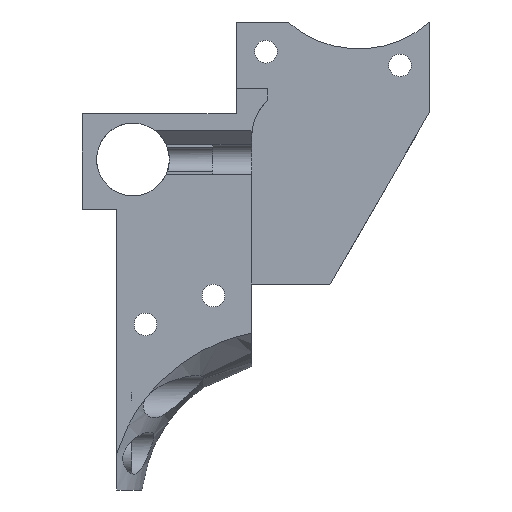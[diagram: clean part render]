
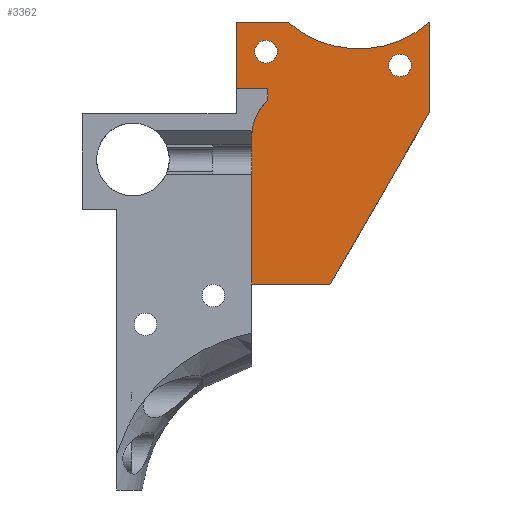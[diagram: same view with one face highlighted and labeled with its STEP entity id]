
A CAD part, left-side view. The second image highlights one B-rep face of the part: STEP entity #3362.
In plain terms, the highlighted planar face has unit normal (-1, 0, 0).
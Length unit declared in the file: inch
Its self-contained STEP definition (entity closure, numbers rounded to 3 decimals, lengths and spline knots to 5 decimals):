
#197=FACE_BOUND('',#874,.T.);
#198=FACE_BOUND('',#875,.T.);
#223=CIRCLE('',#3423,0.25);
#228=CIRCLE('',#3508,0.05906);
#230=CIRCLE('',#3511,0.05906);
#233=CIRCLE('',#3515,0.559);
#675=FACE_OUTER_BOUND('',#873,.T.);
#873=EDGE_LOOP('',(#3140,#3141,#3142,#3143,#3144,#3145,#3146,#3147,#3148,
#3149));
#874=EDGE_LOOP('',(#3150));
#875=EDGE_LOOP('',(#3151));
#914=LINE('',#4498,#1110);
#1031=LINE('',#5590,#1227);
#1041=LINE('',#9068,#1237);
#1048=LINE('',#9093,#1244);
#1049=LINE('',#9095,#1245);
#1068=LINE('',#9408,#1264);
#1070=LINE('',#9411,#1266);
#1071=LINE('',#9413,#1267);
#1110=VECTOR('',#3688,0.3937);
#1227=VECTOR('',#3821,0.3937);
#1237=VECTOR('',#3977,0.3937);
#1244=VECTOR('',#4004,0.3937);
#1245=VECTOR('',#4007,0.3937);
#1264=VECTOR('',#4084,0.3937);
#1266=VECTOR('',#4088,0.3937);
#1267=VECTOR('',#4091,0.3937);
#1325=VERTEX_POINT('',#4483);
#1326=VERTEX_POINT('',#4485);
#1330=VERTEX_POINT('',#4496);
#1551=VERTEX_POINT('',#5587);
#1552=VERTEX_POINT('',#5589);
#1590=VERTEX_POINT('',#9067);
#1591=VERTEX_POINT('',#9071);
#1593=VERTEX_POINT('',#9077);
#1597=VERTEX_POINT('',#9086);
#1598=VERTEX_POINT('',#9088);
#1608=VERTEX_POINT('',#9405);
#1609=VERTEX_POINT('',#9407);
#1683=EDGE_CURVE('',#1326,#1325,#223,.T.);
#1690=EDGE_CURVE('',#1325,#1330,#914,.T.);
#1916=EDGE_CURVE('',#1551,#1552,#1031,.T.);
#2066=EDGE_CURVE('',#1326,#1590,#1041,.T.);
#2068=EDGE_CURVE('',#1591,#1591,#228,.T.);
#2071=EDGE_CURVE('',#1593,#1593,#230,.T.);
#2076=EDGE_CURVE('',#1597,#1598,#233,.T.);
#2079=EDGE_CURVE('',#1552,#1597,#1048,.T.);
#2080=EDGE_CURVE('',#1590,#1551,#1049,.T.);
#2120=EDGE_CURVE('',#1609,#1608,#1068,.T.);
#2122=EDGE_CURVE('',#1330,#1609,#1070,.T.);
#2123=EDGE_CURVE('',#1608,#1598,#1071,.T.);
#3140=ORIENTED_EDGE('',*,*,#1683,.T.);
#3141=ORIENTED_EDGE('',*,*,#1690,.T.);
#3142=ORIENTED_EDGE('',*,*,#2122,.T.);
#3143=ORIENTED_EDGE('',*,*,#2120,.T.);
#3144=ORIENTED_EDGE('',*,*,#2123,.T.);
#3145=ORIENTED_EDGE('',*,*,#2076,.F.);
#3146=ORIENTED_EDGE('',*,*,#2079,.F.);
#3147=ORIENTED_EDGE('',*,*,#1916,.F.);
#3148=ORIENTED_EDGE('',*,*,#2080,.F.);
#3149=ORIENTED_EDGE('',*,*,#2066,.F.);
#3150=ORIENTED_EDGE('',*,*,#2068,.T.);
#3151=ORIENTED_EDGE('',*,*,#2071,.T.);
#3185=PLANE('',#3549);
#3362=ADVANCED_FACE('',(#675,#197,#198),#3185,.T.);
#3423=AXIS2_PLACEMENT_3D('',#4486,#3677,#3678);
#3508=AXIS2_PLACEMENT_3D('',#9072,#3981,#3982);
#3511=AXIS2_PLACEMENT_3D('',#9078,#3988,#3989);
#3515=AXIS2_PLACEMENT_3D('',#9089,#3998,#3999);
#3549=AXIS2_PLACEMENT_3D('',#9414,#4092,#4093);
#3677=DIRECTION('center_axis',(-1.,0.,0.));
#3678=DIRECTION('ref_axis',(0.,0.707,0.707));
#3688=DIRECTION('',(0.,0.,-1.));
#3821=DIRECTION('',(0.,0.,1.));
#3977=DIRECTION('',(0.,0.,1.));
#3981=DIRECTION('center_axis',(1.,0.,0.));
#3982=DIRECTION('ref_axis',(0.,0.,1.));
#3988=DIRECTION('center_axis',(1.,0.,0.));
#3989=DIRECTION('ref_axis',(0.,0.,1.));
#3998=DIRECTION('center_axis',(-1.,0.,0.));
#3999=DIRECTION('ref_axis',(0.,1.,0.));
#4004=DIRECTION('',(0.,-1.,0.));
#4007=DIRECTION('',(0.,1.,0.));
#4084=DIRECTION('',(0.,-0.5,0.866));
#4088=DIRECTION('',(0.,-1.,0.));
#4091=DIRECTION('',(0.,0.,1.));
#4092=DIRECTION('center_axis',(-1.,0.,0.));
#4093=DIRECTION('ref_axis',(0.,0.,1.));
#4483=CARTESIAN_POINT('',(-0.1875,-1.335,-2.188));
#4485=CARTESIAN_POINT('',(-0.1875,-1.4195,-2.00062));
#4486=CARTESIAN_POINT('Origin',(-0.1875,-1.585,-2.188));
#4496=CARTESIAN_POINT('',(-0.1875,-1.335,-2.963));
#4498=CARTESIAN_POINT('',(-0.1875,-1.335,-2.70675));
#5587=CARTESIAN_POINT('',(-0.1875,-1.254,-1.938));
#5589=CARTESIAN_POINT('',(-0.1875,-1.254,-1.59114));
#5590=CARTESIAN_POINT('',(-0.1875,-1.254,-1.85128));
#9067=CARTESIAN_POINT('',(-0.1875,-1.4195,-1.938));
#9068=CARTESIAN_POINT('',(-0.1875,-1.4195,-1.98497));
#9071=CARTESIAN_POINT('',(-0.1875,-1.4095,-1.80541));
#9072=CARTESIAN_POINT('Origin',(-0.1875,-1.4095,-1.74635));
#9077=CARTESIAN_POINT('',(-0.1875,-2.1095,-1.87652));
#9078=CARTESIAN_POINT('Origin',(-0.1875,-2.1095,-1.81746));
#9086=CARTESIAN_POINT('',(-0.1875,-1.523,-1.59114));
#9088=CARTESIAN_POINT('',(-0.1875,-2.265,-1.59114));
#9089=CARTESIAN_POINT('Origin',(-0.1875,-1.894,-1.173));
#9093=CARTESIAN_POINT('',(-0.1875,-1.50675,-1.59114));
#9095=CARTESIAN_POINT('',(-0.1875,-1.50011,-1.938));
#9405=CARTESIAN_POINT('',(-0.1875,-2.265,-2.05992));
#9407=CARTESIAN_POINT('',(-0.1875,-1.74361,-2.963));
#9408=CARTESIAN_POINT('',(-0.1875,-2.12231,-2.30706));
#9411=CARTESIAN_POINT('',(-0.1875,-1.7718,-2.963));
#9413=CARTESIAN_POINT('',(-0.1875,-2.265,-2.19425));
#9414=CARTESIAN_POINT('Origin',(-0.1875,-1.8,-2.4505));
